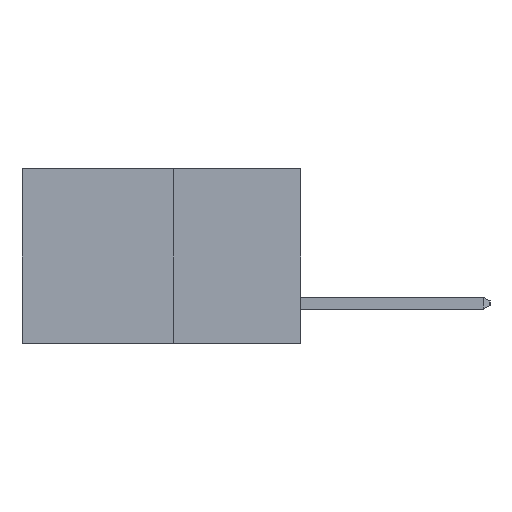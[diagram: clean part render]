
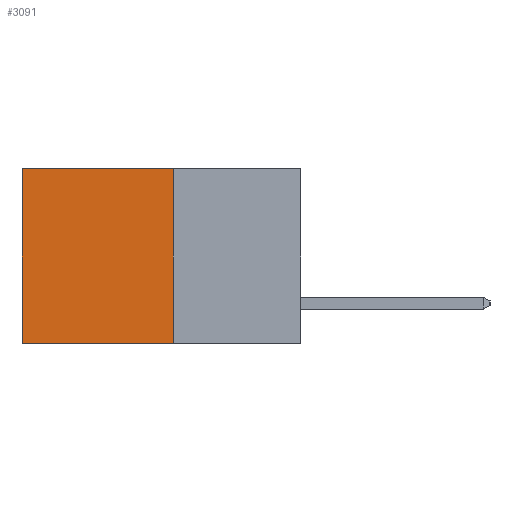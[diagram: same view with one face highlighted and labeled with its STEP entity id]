
A CAD part, left-side view. The second image highlights one B-rep face of the part: STEP entity #3091.
In plain terms, the highlighted planar face has unit normal (-1, 0, 0).
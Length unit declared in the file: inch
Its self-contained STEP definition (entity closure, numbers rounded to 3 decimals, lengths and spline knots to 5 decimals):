
#149 = LINE ( 'NONE', #19150, #21952 ) ;
#280 = ORIENTED_EDGE ( 'NONE', *, *, #3195, .T. ) ;
#1392 = AXIS2_PLACEMENT_3D ( 'NONE', #5172, #7268, #21940 ) ;
#3091 = ADVANCED_FACE ( 'NONE', ( #23232 ), #19821, .F. ) ;
#3195 = EDGE_CURVE ( 'NONE', #12125, #19794, #25488, .T. ) ;
#5172 = CARTESIAN_POINT ( 'NONE',  ( 0.277, 0.27, -0.37 ) ) ;
#5221 = ORIENTED_EDGE ( 'NONE', *, *, #21021, .T. ) ;
#7268 = DIRECTION ( 'NONE',  ( 1., 0., 0. ) ) ;
#7846 = CARTESIAN_POINT ( 'NONE',  ( 0.277, 0.27, -0.37 ) ) ;
#9378 = CARTESIAN_POINT ( 'NONE',  ( 0.277, 0.27, -0.37 ) ) ;
#9885 = LINE ( 'NONE', #7846, #19738 ) ;
#10487 = EDGE_CURVE ( 'NONE', #10924, #18092, #21727, .T. ) ;
#10924 = VERTEX_POINT ( 'NONE', #20972 ) ;
#12125 = VERTEX_POINT ( 'NONE', #18317 ) ;
#13809 = DIRECTION ( 'NONE',  ( 0., 0., -1. ) ) ;
#14300 = VECTOR ( 'NONE', #13809, 39.37008 ) ;
#16974 = CARTESIAN_POINT ( 'NONE',  ( 0.277, 0.59, -0.37 ) ) ;
#17304 = CARTESIAN_POINT ( 'NONE',  ( 0.277, 0.27, -0.37 ) ) ;
#18092 = VERTEX_POINT ( 'NONE', #9378 ) ;
#18317 = CARTESIAN_POINT ( 'NONE',  ( 0.277, 0.59, 0. ) ) ;
#19150 = CARTESIAN_POINT ( 'NONE',  ( 0.277, 0.27, 0. ) ) ;
#19587 = EDGE_CURVE ( 'NONE', #18092, #19794, #9885, .T. ) ;
#19738 = VECTOR ( 'NONE', #24622, 39.37008 ) ;
#19794 = VERTEX_POINT ( 'NONE', #16974 ) ;
#19821 = PLANE ( 'NONE',  #1392 ) ;
#20972 = CARTESIAN_POINT ( 'NONE',  ( 0.277, 0.27, 0. ) ) ;
#21021 = EDGE_CURVE ( 'NONE', #10924, #12125, #149, .T. ) ;
#21080 = VECTOR ( 'NONE', #25739, 39.37008 ) ;
#21276 = DIRECTION ( 'NONE',  ( 0., 1., 0. ) ) ;
#21727 = LINE ( 'NONE', #17304, #21080 ) ;
#21940 = DIRECTION ( 'NONE',  ( 0., 0., -1. ) ) ;
#21952 = VECTOR ( 'NONE', #21276, 39.37008 ) ;
#23232 = FACE_OUTER_BOUND ( 'NONE', #24626, .T. ) ;
#24311 = CARTESIAN_POINT ( 'NONE',  ( 0.277, 0.59, -0.37 ) ) ;
#24622 = DIRECTION ( 'NONE',  ( 0., 1., 0. ) ) ;
#24626 = EDGE_LOOP ( 'NONE', ( #280, #24967, #25916, #5221 ) ) ;
#24967 = ORIENTED_EDGE ( 'NONE', *, *, #19587, .F. ) ;
#25488 = LINE ( 'NONE', #24311, #14300 ) ;
#25739 = DIRECTION ( 'NONE',  ( 0., 0., -1. ) ) ;
#25916 = ORIENTED_EDGE ( 'NONE', *, *, #10487, .F. ) ;
